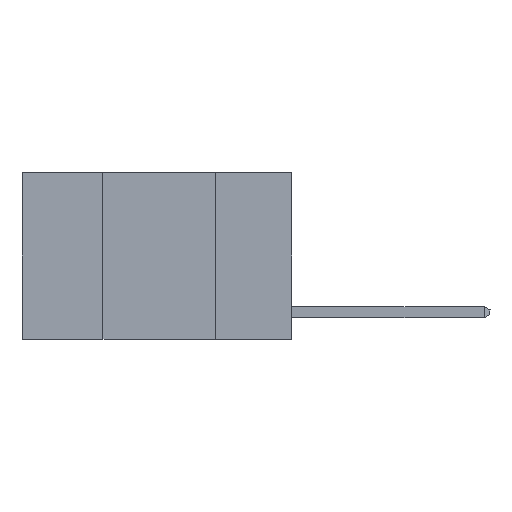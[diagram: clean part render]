
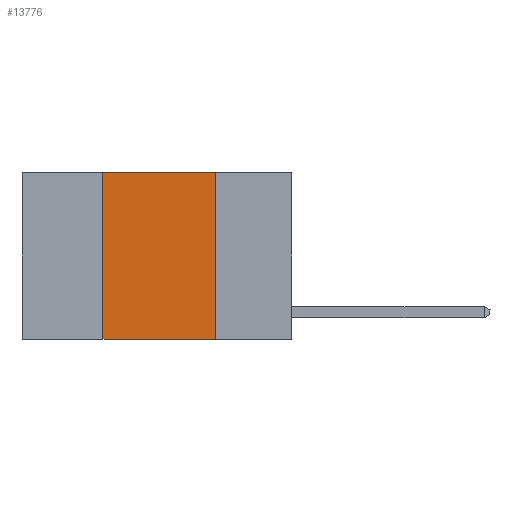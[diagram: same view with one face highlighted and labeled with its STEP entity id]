
A CAD part, left-side view. The second image highlights one B-rep face of the part: STEP entity #13776.
In plain terms, the highlighted planar face has unit normal (-1, 0, 0).
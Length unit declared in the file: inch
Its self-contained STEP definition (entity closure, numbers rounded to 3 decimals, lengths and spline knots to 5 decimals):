
#957 = LINE ( 'NONE', #4957, #16379 ) ;
#1224 = DIRECTION ( 'NONE',  ( 1., 0., 0. ) ) ;
#1864 = EDGE_CURVE ( 'NONE', #16056, #16509, #14295, .T. ) ;
#1996 = EDGE_LOOP ( 'NONE', ( #3082, #4241, #8167, #4017 ) ) ;
#2147 = CARTESIAN_POINT ( 'NONE',  ( 0., 0.17, -0.37 ) ) ;
#2357 = FACE_OUTER_BOUND ( 'NONE', #1996, .T. ) ;
#2723 = EDGE_CURVE ( 'NONE', #5909, #15109, #957, .T. ) ;
#2753 = CARTESIAN_POINT ( 'NONE',  ( 0., 0.17, 0. ) ) ;
#3082 = ORIENTED_EDGE ( 'NONE', *, *, #1864, .F. ) ;
#4017 = ORIENTED_EDGE ( 'NONE', *, *, #17001, .T. ) ;
#4241 = ORIENTED_EDGE ( 'NONE', *, *, #15822, .F. ) ;
#4957 = CARTESIAN_POINT ( 'NONE',  ( 0., 0.42, 0. ) ) ;
#5909 = VERTEX_POINT ( 'NONE', #12929 ) ;
#6079 = DIRECTION ( 'NONE',  ( 0., -1., 0. ) ) ;
#6300 = AXIS2_PLACEMENT_3D ( 'NONE', #13163, #1224, #12052 ) ;
#6672 = LINE ( 'NONE', #11361, #14939 ) ;
#7269 = CARTESIAN_POINT ( 'NONE',  ( 0., 0.6, -0.37 ) ) ;
#7800 = DIRECTION ( 'NONE',  ( 0., 0., 1. ) ) ;
#8167 = ORIENTED_EDGE ( 'NONE', *, *, #2723, .F. ) ;
#9335 = CARTESIAN_POINT ( 'NONE',  ( 0., 0.17, 0. ) ) ;
#10300 = PLANE ( 'NONE',  #6300 ) ;
#10304 = LINE ( 'NONE', #7269, #10949 ) ;
#10949 = VECTOR ( 'NONE', #6079, 39.37008 ) ;
#11173 = VECTOR ( 'NONE', #11962, 39.37008 ) ;
#11361 = CARTESIAN_POINT ( 'NONE',  ( 0., 0.6, 0. ) ) ;
#11962 = DIRECTION ( 'NONE',  ( 0., 0., -1. ) ) ;
#12052 = DIRECTION ( 'NONE',  ( 0., 0., -1. ) ) ;
#12415 = CARTESIAN_POINT ( 'NONE',  ( 0., 0.42, 0. ) ) ;
#12929 = CARTESIAN_POINT ( 'NONE',  ( 0., 0.42, -0.37 ) ) ;
#13163 = CARTESIAN_POINT ( 'NONE',  ( 0., 0.6, 0. ) ) ;
#13776 = ADVANCED_FACE ( 'NONE', ( #2357 ), #10300, .F. ) ;
#14042 = DIRECTION ( 'NONE',  ( 0., -1., 0. ) ) ;
#14295 = LINE ( 'NONE', #9335, #11173 ) ;
#14939 = VECTOR ( 'NONE', #14042, 39.37008 ) ;
#15109 = VERTEX_POINT ( 'NONE', #12415 ) ;
#15822 = EDGE_CURVE ( 'NONE', #15109, #16056, #6672, .T. ) ;
#16056 = VERTEX_POINT ( 'NONE', #2753 ) ;
#16379 = VECTOR ( 'NONE', #7800, 39.37008 ) ;
#16509 = VERTEX_POINT ( 'NONE', #2147 ) ;
#17001 = EDGE_CURVE ( 'NONE', #5909, #16509, #10304, .T. ) ;
